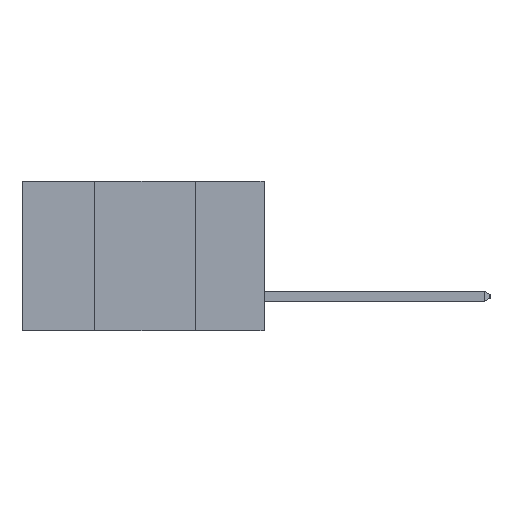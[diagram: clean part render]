
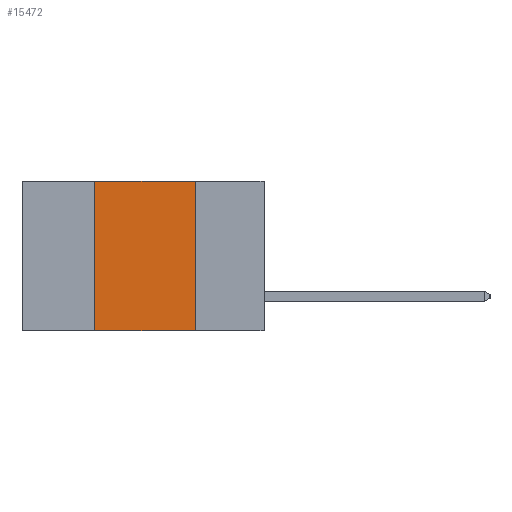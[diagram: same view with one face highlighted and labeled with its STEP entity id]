
A CAD part, left-side view. The second image highlights one B-rep face of the part: STEP entity #15472.
In plain terms, the highlighted planar face has unit normal (-1, 0, 0).
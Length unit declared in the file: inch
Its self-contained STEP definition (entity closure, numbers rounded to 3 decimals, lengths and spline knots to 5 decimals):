
#161 = CARTESIAN_POINT ( 'NONE',  ( 0., 0.6, -0.37 ) ) ;
#376 = VECTOR ( 'NONE', #9153, 39.37008 ) ;
#656 = ORIENTED_EDGE ( 'NONE', *, *, #6871, .F. ) ;
#930 = VERTEX_POINT ( 'NONE', #3438 ) ;
#976 = DIRECTION ( 'NONE',  ( 0., 0., -1. ) ) ;
#2028 = ORIENTED_EDGE ( 'NONE', *, *, #8494, .F. ) ;
#2804 = DIRECTION ( 'NONE',  ( 0., -1., 0. ) ) ;
#3076 = CARTESIAN_POINT ( 'NONE',  ( 0., 0.17, 0. ) ) ;
#3146 = CARTESIAN_POINT ( 'NONE',  ( 0., 0.6, 0. ) ) ;
#3438 = CARTESIAN_POINT ( 'NONE',  ( 0., 0.17, -0.37 ) ) ;
#3548 = VECTOR ( 'NONE', #6174, 39.37008 ) ;
#4028 = LINE ( 'NONE', #161, #3548 ) ;
#5043 = CARTESIAN_POINT ( 'NONE',  ( 0., 0.42, -0.37 ) ) ;
#6174 = DIRECTION ( 'NONE',  ( 0., -1., 0. ) ) ;
#6731 = VECTOR ( 'NONE', #2804, 39.37008 ) ;
#6737 = ORIENTED_EDGE ( 'NONE', *, *, #13257, .T. ) ;
#6871 = EDGE_CURVE ( 'NONE', #16626, #930, #12176, .T. ) ;
#7864 = EDGE_CURVE ( 'NONE', #13802, #16626, #17926, .T. ) ;
#8143 = VECTOR ( 'NONE', #15289, 39.37008 ) ;
#8445 = PLANE ( 'NONE',  #11404 ) ;
#8494 = EDGE_CURVE ( 'NONE', #16861, #13802, #15639, .T. ) ;
#8976 = CARTESIAN_POINT ( 'NONE',  ( 0., 0.17, -0.37 ) ) ;
#9153 = DIRECTION ( 'NONE',  ( 0., 0., -1. ) ) ;
#9209 = CARTESIAN_POINT ( 'NONE',  ( 0., 0.42, 0. ) ) ;
#9924 = DIRECTION ( 'NONE',  ( 1., 0., 0. ) ) ;
#11404 = AXIS2_PLACEMENT_3D ( 'NONE', #16812, #9924, #976 ) ;
#12176 = LINE ( 'NONE', #8976, #376 ) ;
#13257 = EDGE_CURVE ( 'NONE', #16861, #930, #4028, .T. ) ;
#13802 = VERTEX_POINT ( 'NONE', #9209 ) ;
#15289 = DIRECTION ( 'NONE',  ( 0., 0., 1. ) ) ;
#15311 = CARTESIAN_POINT ( 'NONE',  ( 0., 0.42, -0.37 ) ) ;
#15472 = ADVANCED_FACE ( 'NONE', ( #15879 ), #8445, .F. ) ;
#15639 = LINE ( 'NONE', #15311, #8143 ) ;
#15879 = FACE_OUTER_BOUND ( 'NONE', #17783, .T. ) ;
#16626 = VERTEX_POINT ( 'NONE', #3076 ) ;
#16732 = ORIENTED_EDGE ( 'NONE', *, *, #7864, .F. ) ;
#16812 = CARTESIAN_POINT ( 'NONE',  ( 0., 0.6, 0. ) ) ;
#16861 = VERTEX_POINT ( 'NONE', #5043 ) ;
#17783 = EDGE_LOOP ( 'NONE', ( #656, #16732, #2028, #6737 ) ) ;
#17926 = LINE ( 'NONE', #3146, #6731 ) ;
